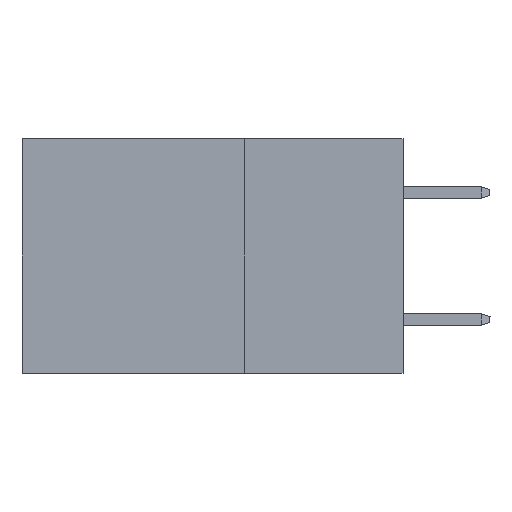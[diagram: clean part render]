
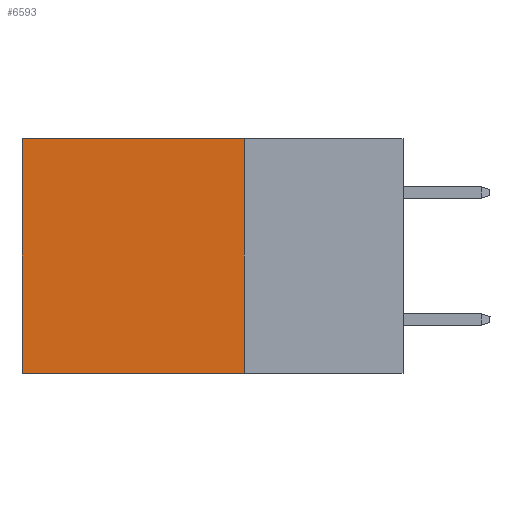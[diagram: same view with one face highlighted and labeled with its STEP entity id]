
A CAD part, left-side view. The second image highlights one B-rep face of the part: STEP entity #6593.
In plain terms, the highlighted planar face has unit normal (-1, 0, 0).
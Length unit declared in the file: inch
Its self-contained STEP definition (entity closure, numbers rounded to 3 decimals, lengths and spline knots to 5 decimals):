
#52 = CARTESIAN_POINT ( 'NONE',  ( 0.2875, 0.25, 0. ) ) ;
#616 = EDGE_CURVE ( 'NONE', #1397, #3911, #12586, .T. ) ;
#640 = VECTOR ( 'NONE', #11928, 39.37008 ) ;
#1165 = LINE ( 'NONE', #10726, #8160 ) ;
#1218 = ORIENTED_EDGE ( 'NONE', *, *, #616, .F. ) ;
#1346 = VECTOR ( 'NONE', #10025, 39.37008 ) ;
#1373 = ORIENTED_EDGE ( 'NONE', *, *, #4911, .T. ) ;
#1397 = VERTEX_POINT ( 'NONE', #7764 ) ;
#1402 = ORIENTED_EDGE ( 'NONE', *, *, #2864, .F. ) ;
#1435 = DIRECTION ( 'NONE',  ( 0., 1., 0. ) ) ;
#1896 = PLANE ( 'NONE',  #2119 ) ;
#2119 = AXIS2_PLACEMENT_3D ( 'NONE', #52, #11401, #13369 ) ;
#2864 = EDGE_CURVE ( 'NONE', #3911, #8176, #1165, .T. ) ;
#3540 = CARTESIAN_POINT ( 'NONE',  ( 0.2875, 0.6, -0.37 ) ) ;
#3911 = VERTEX_POINT ( 'NONE', #12855 ) ;
#4911 = EDGE_CURVE ( 'NONE', #1397, #9958, #12813, .T. ) ;
#5255 = ORIENTED_EDGE ( 'NONE', *, *, #9067, .T. ) ;
#5578 = DIRECTION ( 'NONE',  ( 0., 0., -1. ) ) ;
#5764 = CARTESIAN_POINT ( 'NONE',  ( 0.2875, 0.25, 0. ) ) ;
#6565 = CARTESIAN_POINT ( 'NONE',  ( 0.2875, 0.6, 0. ) ) ;
#6593 = ADVANCED_FACE ( 'NONE', ( #8776 ), #1896, .F. ) ;
#6785 = EDGE_LOOP ( 'NONE', ( #5255, #1402, #1218, #1373 ) ) ;
#7764 = CARTESIAN_POINT ( 'NONE',  ( 0.2875, 0.25, 0. ) ) ;
#8160 = VECTOR ( 'NONE', #1435, 39.37008 ) ;
#8176 = VERTEX_POINT ( 'NONE', #3540 ) ;
#8776 = FACE_OUTER_BOUND ( 'NONE', #6785, .T. ) ;
#9067 = EDGE_CURVE ( 'NONE', #9958, #8176, #9839, .T. ) ;
#9839 = LINE ( 'NONE', #6565, #11152 ) ;
#9958 = VERTEX_POINT ( 'NONE', #11212 ) ;
#10025 = DIRECTION ( 'NONE',  ( 0., 0., -1. ) ) ;
#10726 = CARTESIAN_POINT ( 'NONE',  ( 0.2875, 0.25, -0.37 ) ) ;
#11152 = VECTOR ( 'NONE', #5578, 39.37008 ) ;
#11212 = CARTESIAN_POINT ( 'NONE',  ( 0.2875, 0.6, 0. ) ) ;
#11401 = DIRECTION ( 'NONE',  ( 1., 0., 0. ) ) ;
#11928 = DIRECTION ( 'NONE',  ( 0., 1., 0. ) ) ;
#12586 = LINE ( 'NONE', #5764, #1346 ) ;
#12813 = LINE ( 'NONE', #12875, #640 ) ;
#12855 = CARTESIAN_POINT ( 'NONE',  ( 0.2875, 0.25, -0.37 ) ) ;
#12875 = CARTESIAN_POINT ( 'NONE',  ( 0.2875, 0.25, 0. ) ) ;
#13369 = DIRECTION ( 'NONE',  ( 0., 0., -1. ) ) ;
